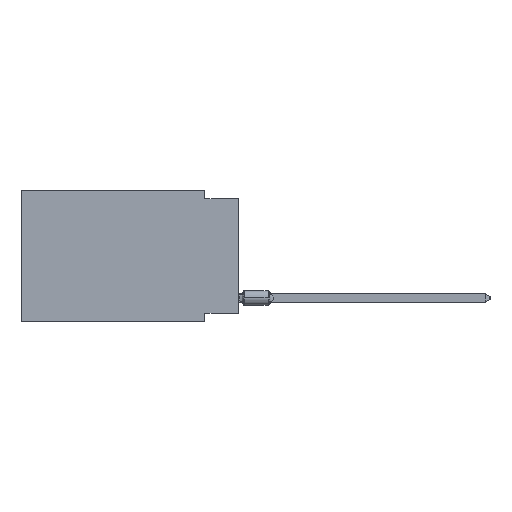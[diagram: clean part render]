
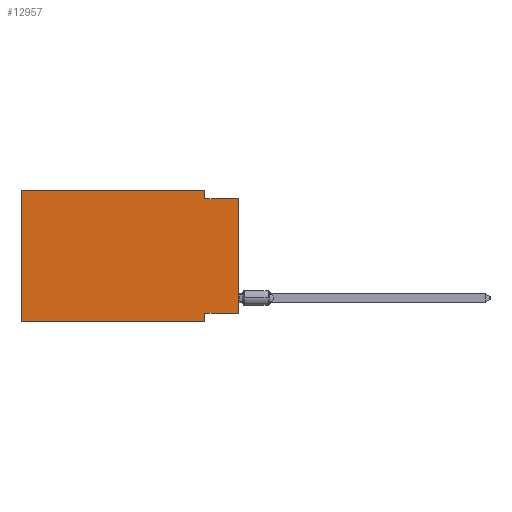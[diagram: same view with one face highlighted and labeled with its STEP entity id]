
A CAD part, left-side view. The second image highlights one B-rep face of the part: STEP entity #12957.
In plain terms, the highlighted planar face has unit normal (-1, 0, 0).
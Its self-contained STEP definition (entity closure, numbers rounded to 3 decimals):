
#381 = CARTESIAN_POINT ( 'NONE',  ( 0., 16.383, 0. ) ) ;
#903 = CARTESIAN_POINT ( 'NONE',  ( 0., 2.54, 0. ) ) ;
#1365 = ORIENTED_EDGE ( 'NONE', *, *, #52317, .F. ) ;
#1432 = VECTOR ( 'NONE', #14960, 1000. ) ;
#1845 = CARTESIAN_POINT ( 'NONE',  ( 0., 16.383, 0. ) ) ;
#4280 = CARTESIAN_POINT ( 'NONE',  ( 0., 2.54, 0. ) ) ;
#6558 = DIRECTION ( 'NONE',  ( 0., -1., 0. ) ) ;
#7070 = CARTESIAN_POINT ( 'NONE',  ( 0., 0., -0.635 ) ) ;
#7280 = VERTEX_POINT ( 'NONE', #13574 ) ;
#7796 = ORIENTED_EDGE ( 'NONE', *, *, #10854, .T. ) ;
#8978 = VERTEX_POINT ( 'NONE', #15493 ) ;
#9653 = EDGE_CURVE ( 'NONE', #49469, #26260, #51867, .T. ) ;
#10854 = EDGE_CURVE ( 'NONE', #44463, #20037, #16530, .T. ) ;
#10970 = VECTOR ( 'NONE', #50457, 1000. ) ;
#12740 = CARTESIAN_POINT ( 'NONE',  ( 0., 2.54, -9.906 ) ) ;
#12916 = VERTEX_POINT ( 'NONE', #4280 ) ;
#12928 = CARTESIAN_POINT ( 'NONE',  ( 0., 0., -9.271 ) ) ;
#12957 = ADVANCED_FACE ( 'NONE', ( #39794 ), #21665, .F. ) ;
#13574 = CARTESIAN_POINT ( 'NONE',  ( 0., 2.54, -9.906 ) ) ;
#14437 = VECTOR ( 'NONE', #6558, 1000. ) ;
#14718 = LINE ( 'NONE', #1845, #47991 ) ;
#14903 = VERTEX_POINT ( 'NONE', #47091 ) ;
#14960 = DIRECTION ( 'NONE',  ( 0., -1., 0. ) ) ;
#14992 = CARTESIAN_POINT ( 'NONE',  ( 0., 16.383, -9.906 ) ) ;
#15234 = VECTOR ( 'NONE', #43503, 1000. ) ;
#15493 = CARTESIAN_POINT ( 'NONE',  ( 0., 2.54, -9.271 ) ) ;
#16530 = LINE ( 'NONE', #29904, #52059 ) ;
#18109 = EDGE_CURVE ( 'NONE', #49469, #7280, #40686, .T. ) ;
#18253 = DIRECTION ( 'NONE',  ( 0., 1., 0. ) ) ;
#18670 = EDGE_CURVE ( 'NONE', #44463, #8978, #22178, .T. ) ;
#18807 = ORIENTED_EDGE ( 'NONE', *, *, #18670, .F. ) ;
#18926 = EDGE_LOOP ( 'NONE', ( #7796, #32742, #1365, #35453, #24604, #45014, #51539, #18807 ) ) ;
#20037 = VERTEX_POINT ( 'NONE', #46659 ) ;
#21665 = PLANE ( 'NONE',  #36234 ) ;
#21834 = DIRECTION ( 'NONE',  ( 0., 0., 1. ) ) ;
#21916 = LINE ( 'NONE', #903, #48769 ) ;
#22178 = LINE ( 'NONE', #12928, #25044 ) ;
#23006 = CARTESIAN_POINT ( 'NONE',  ( 0., 16.383, 0. ) ) ;
#24604 = ORIENTED_EDGE ( 'NONE', *, *, #9653, .F. ) ;
#25044 = VECTOR ( 'NONE', #18253, 1000. ) ;
#26260 = VERTEX_POINT ( 'NONE', #23006 ) ;
#29027 = CARTESIAN_POINT ( 'NONE',  ( 0., 16.383, -9.906 ) ) ;
#29904 = CARTESIAN_POINT ( 'NONE',  ( 0., 0., 0. ) ) ;
#32564 = EDGE_CURVE ( 'NONE', #26260, #12916, #14718, .T. ) ;
#32742 = ORIENTED_EDGE ( 'NONE', *, *, #52064, .F. ) ;
#34768 = DIRECTION ( 'NONE',  ( 0., 0., -1. ) ) ;
#35453 = ORIENTED_EDGE ( 'NONE', *, *, #32564, .F. ) ;
#36142 = CARTESIAN_POINT ( 'NONE',  ( 0., 0., -9.271 ) ) ;
#36234 = AXIS2_PLACEMENT_3D ( 'NONE', #381, #52603, #34768 ) ;
#39794 = FACE_OUTER_BOUND ( 'NONE', #18926, .T. ) ;
#40686 = LINE ( 'NONE', #14992, #14437 ) ;
#40926 = LINE ( 'NONE', #7070, #1432 ) ;
#41807 = LINE ( 'NONE', #12740, #10970 ) ;
#42396 = CARTESIAN_POINT ( 'NONE',  ( 0., 16.383, 0. ) ) ;
#43503 = DIRECTION ( 'NONE',  ( 0., 0., 1. ) ) ;
#44463 = VERTEX_POINT ( 'NONE', #36142 ) ;
#45014 = ORIENTED_EDGE ( 'NONE', *, *, #18109, .T. ) ;
#46659 = CARTESIAN_POINT ( 'NONE',  ( 0., 0., -0.635 ) ) ;
#47091 = CARTESIAN_POINT ( 'NONE',  ( 0., 2.54, -0.635 ) ) ;
#47859 = DIRECTION ( 'NONE',  ( 0., 0., -1. ) ) ;
#47991 = VECTOR ( 'NONE', #53229, 1000. ) ;
#48769 = VECTOR ( 'NONE', #47859, 1000. ) ;
#49469 = VERTEX_POINT ( 'NONE', #29027 ) ;
#50457 = DIRECTION ( 'NONE',  ( 0., 0., -1. ) ) ;
#50642 = EDGE_CURVE ( 'NONE', #8978, #7280, #41807, .T. ) ;
#51539 = ORIENTED_EDGE ( 'NONE', *, *, #50642, .F. ) ;
#51867 = LINE ( 'NONE', #42396, #15234 ) ;
#52059 = VECTOR ( 'NONE', #21834, 1000. ) ;
#52064 = EDGE_CURVE ( 'NONE', #14903, #20037, #40926, .T. ) ;
#52317 = EDGE_CURVE ( 'NONE', #12916, #14903, #21916, .T. ) ;
#52603 = DIRECTION ( 'NONE',  ( 1., 0., 0. ) ) ;
#53229 = DIRECTION ( 'NONE',  ( 0., -1., 0. ) ) ;
